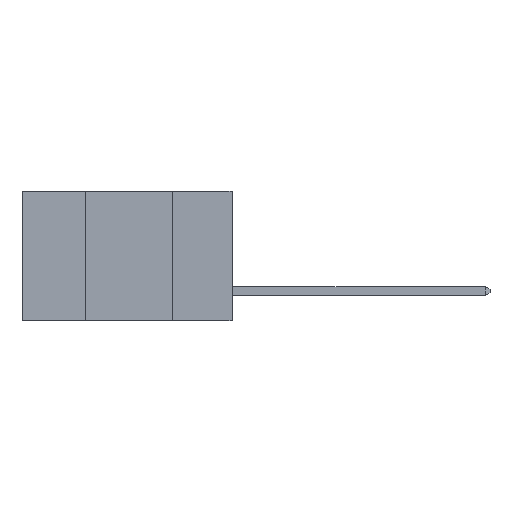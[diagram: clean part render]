
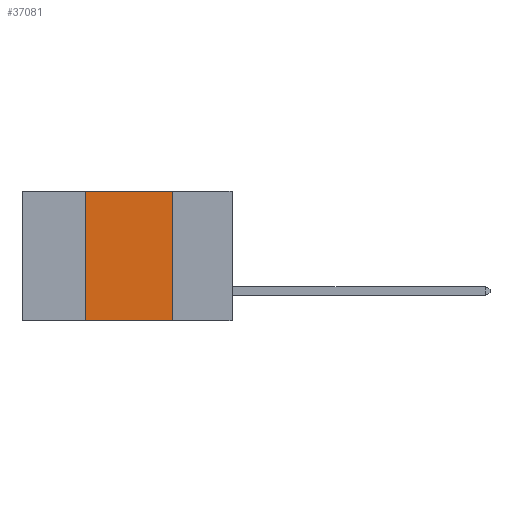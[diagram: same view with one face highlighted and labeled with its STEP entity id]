
A CAD part, left-side view. The second image highlights one B-rep face of the part: STEP entity #37081.
In plain terms, the highlighted planar face has unit normal (-1, 0, 0).
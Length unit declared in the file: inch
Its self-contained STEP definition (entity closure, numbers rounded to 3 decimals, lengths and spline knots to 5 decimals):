
#503 = CARTESIAN_POINT ( 'NONE',  ( 0., 0.6, 0. ) ) ;
#629 = DIRECTION ( 'NONE',  ( 1., 0., 0. ) ) ;
#1578 = EDGE_CURVE ( 'NONE', #5226, #27658, #11424, .T. ) ;
#1940 = CARTESIAN_POINT ( 'NONE',  ( 0., 0.42, 0. ) ) ;
#2201 = ORIENTED_EDGE ( 'NONE', *, *, #19768, .F. ) ;
#2738 = VECTOR ( 'NONE', #15140, 39.37008 ) ;
#2777 = CARTESIAN_POINT ( 'NONE',  ( 0., 0.17, -0.37 ) ) ;
#3517 = PLANE ( 'NONE',  #6118 ) ;
#4690 = LINE ( 'NONE', #12954, #27060 ) ;
#5226 = VERTEX_POINT ( 'NONE', #37382 ) ;
#6118 = AXIS2_PLACEMENT_3D ( 'NONE', #503, #629, #21170 ) ;
#8423 = CARTESIAN_POINT ( 'NONE',  ( 0., 0.6, -0.37 ) ) ;
#8444 = ORIENTED_EDGE ( 'NONE', *, *, #33229, .F. ) ;
#9194 = ORIENTED_EDGE ( 'NONE', *, *, #28954, .T. ) ;
#10068 = VECTOR ( 'NONE', #34514, 39.37008 ) ;
#10657 = CARTESIAN_POINT ( 'NONE',  ( 0., 0.17, 0. ) ) ;
#11258 = CARTESIAN_POINT ( 'NONE',  ( 0., 0.6, 0. ) ) ;
#11424 = LINE ( 'NONE', #20938, #2738 ) ;
#12678 = ORIENTED_EDGE ( 'NONE', *, *, #1578, .F. ) ;
#12954 = CARTESIAN_POINT ( 'NONE',  ( 0., 0.17, 0. ) ) ;
#15140 = DIRECTION ( 'NONE',  ( 0., 0., 1. ) ) ;
#15205 = LINE ( 'NONE', #8423, #29766 ) ;
#17004 = VERTEX_POINT ( 'NONE', #2777 ) ;
#17839 = LINE ( 'NONE', #11258, #10068 ) ;
#19768 = EDGE_CURVE ( 'NONE', #25241, #17004, #4690, .T. ) ;
#20175 = DIRECTION ( 'NONE',  ( 0., -1., 0. ) ) ;
#20938 = CARTESIAN_POINT ( 'NONE',  ( 0., 0.42, 0. ) ) ;
#21170 = DIRECTION ( 'NONE',  ( 0., 0., -1. ) ) ;
#25241 = VERTEX_POINT ( 'NONE', #10657 ) ;
#27060 = VECTOR ( 'NONE', #36332, 39.37008 ) ;
#27658 = VERTEX_POINT ( 'NONE', #1940 ) ;
#28954 = EDGE_CURVE ( 'NONE', #5226, #17004, #15205, .T. ) ;
#29766 = VECTOR ( 'NONE', #20175, 39.37008 ) ;
#31119 = FACE_OUTER_BOUND ( 'NONE', #34312, .T. ) ;
#33229 = EDGE_CURVE ( 'NONE', #27658, #25241, #17839, .T. ) ;
#34312 = EDGE_LOOP ( 'NONE', ( #2201, #8444, #12678, #9194 ) ) ;
#34514 = DIRECTION ( 'NONE',  ( 0., -1., 0. ) ) ;
#36332 = DIRECTION ( 'NONE',  ( 0., 0., -1. ) ) ;
#37081 = ADVANCED_FACE ( 'NONE', ( #31119 ), #3517, .F. ) ;
#37382 = CARTESIAN_POINT ( 'NONE',  ( 0., 0.42, -0.37 ) ) ;
